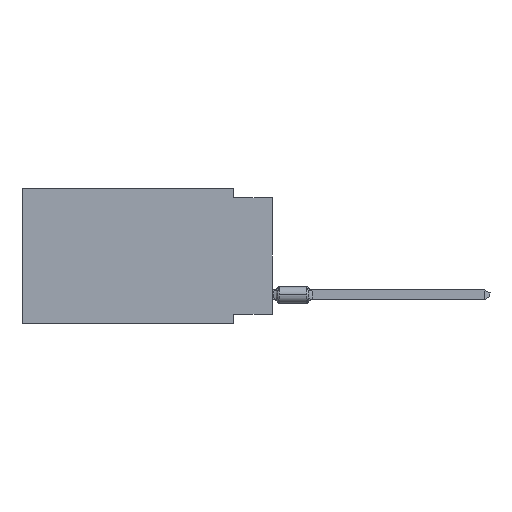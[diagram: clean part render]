
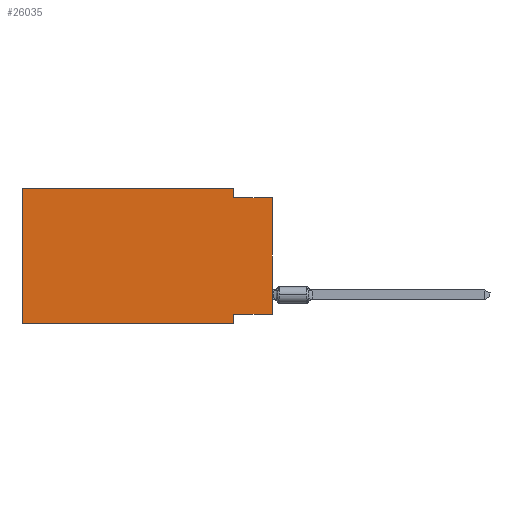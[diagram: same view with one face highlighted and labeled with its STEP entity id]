
A CAD part, left-side view. The second image highlights one B-rep face of the part: STEP entity #26035.
In plain terms, the highlighted planar face has unit normal (-1, 0, 0).
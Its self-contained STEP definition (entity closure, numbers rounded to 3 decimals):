
#2601 = CARTESIAN_POINT ( 'NONE',  ( 0., 16.383, 0. ) ) ;
#3043 = DIRECTION ( 'NONE',  ( 0., 0., 1. ) ) ;
#3452 = DIRECTION ( 'NONE',  ( 0., -1., 0. ) ) ;
#3476 = LINE ( 'NONE', #7590, #48642 ) ;
#3518 = LINE ( 'NONE', #36686, #8659 ) ;
#3585 = VERTEX_POINT ( 'NONE', #44069 ) ;
#4729 = VERTEX_POINT ( 'NONE', #6544 ) ;
#5731 = ORIENTED_EDGE ( 'NONE', *, *, #37576, .F. ) ;
#6544 = CARTESIAN_POINT ( 'NONE',  ( 0., 16.383, -8.89 ) ) ;
#6561 = AXIS2_PLACEMENT_3D ( 'NONE', #48879, #20068, #49409 ) ;
#7590 = CARTESIAN_POINT ( 'NONE',  ( 0., 16.383, -8.89 ) ) ;
#7794 = LINE ( 'NONE', #2601, #51098 ) ;
#8154 = ORIENTED_EDGE ( 'NONE', *, *, #47848, .F. ) ;
#8659 = VECTOR ( 'NONE', #41069, 1000. ) ;
#9269 = ORIENTED_EDGE ( 'NONE', *, *, #39718, .F. ) ;
#9792 = LINE ( 'NONE', #44754, #15389 ) ;
#10535 = ORIENTED_EDGE ( 'NONE', *, *, #14698, .F. ) ;
#11265 = LINE ( 'NONE', #19460, #43617 ) ;
#11359 = DIRECTION ( 'NONE',  ( 0., -1., 0. ) ) ;
#11933 = CARTESIAN_POINT ( 'NONE',  ( 0., 0., -0.635 ) ) ;
#14216 = VERTEX_POINT ( 'NONE', #29497 ) ;
#14698 = EDGE_CURVE ( 'NONE', #32085, #25945, #36820, .T. ) ;
#14884 = DIRECTION ( 'NONE',  ( 0., 0., -1. ) ) ;
#15023 = ORIENTED_EDGE ( 'NONE', *, *, #52276, .F. ) ;
#15389 = VECTOR ( 'NONE', #14884, 1000. ) ;
#16014 = CARTESIAN_POINT ( 'NONE',  ( 0., 2.54, -8.89 ) ) ;
#16252 = ORIENTED_EDGE ( 'NONE', *, *, #40218, .F. ) ;
#17627 = DIRECTION ( 'NONE',  ( 0., 0., 1. ) ) ;
#17725 = VECTOR ( 'NONE', #29119, 1000. ) ;
#19460 = CARTESIAN_POINT ( 'NONE',  ( 0., 16.383, 0. ) ) ;
#19691 = ORIENTED_EDGE ( 'NONE', *, *, #44453, .T. ) ;
#20068 = DIRECTION ( 'NONE',  ( 1., 0., 0. ) ) ;
#20894 = VERTEX_POINT ( 'NONE', #16014 ) ;
#22002 = LINE ( 'NONE', #51358, #38965 ) ;
#22058 = VERTEX_POINT ( 'NONE', #44297 ) ;
#23468 = ORIENTED_EDGE ( 'NONE', *, *, #46355, .T. ) ;
#24189 = VECTOR ( 'NONE', #3452, 1000. ) ;
#24281 = LINE ( 'NONE', #11933, #24189 ) ;
#24557 = DIRECTION ( 'NONE',  ( 0., -1., 0. ) ) ;
#25945 = VERTEX_POINT ( 'NONE', #52438 ) ;
#26035 = ADVANCED_FACE ( 'NONE', ( #40641 ), #53253, .F. ) ;
#26358 = CARTESIAN_POINT ( 'NONE',  ( 0., 2.54, 0. ) ) ;
#27156 = VERTEX_POINT ( 'NONE', #53345 ) ;
#29119 = DIRECTION ( 'NONE',  ( 0., 0., -1. ) ) ;
#29497 = CARTESIAN_POINT ( 'NONE',  ( 0., 2.54, -8.255 ) ) ;
#32085 = VERTEX_POINT ( 'NONE', #26358 ) ;
#36686 = CARTESIAN_POINT ( 'NONE',  ( 0., 0., -8.255 ) ) ;
#36820 = LINE ( 'NONE', #37627, #17725 ) ;
#37576 = EDGE_CURVE ( 'NONE', #25945, #22058, #24281, .T. ) ;
#37627 = CARTESIAN_POINT ( 'NONE',  ( 0., 2.54, 0. ) ) ;
#38965 = VECTOR ( 'NONE', #17627, 1000. ) ;
#39718 = EDGE_CURVE ( 'NONE', #4729, #3585, #11265, .T. ) ;
#40218 = EDGE_CURVE ( 'NONE', #27156, #14216, #3518, .T. ) ;
#40641 = FACE_OUTER_BOUND ( 'NONE', #43732, .T. ) ;
#41069 = DIRECTION ( 'NONE',  ( 0., 1., 0. ) ) ;
#43617 = VECTOR ( 'NONE', #3043, 1000. ) ;
#43732 = EDGE_LOOP ( 'NONE', ( #19691, #5731, #10535, #8154, #9269, #23468, #15023, #16252 ) ) ;
#44069 = CARTESIAN_POINT ( 'NONE',  ( 0., 16.383, 0. ) ) ;
#44297 = CARTESIAN_POINT ( 'NONE',  ( 0., 0., -0.635 ) ) ;
#44453 = EDGE_CURVE ( 'NONE', #27156, #22058, #22002, .T. ) ;
#44754 = CARTESIAN_POINT ( 'NONE',  ( 0., 2.54, -8.89 ) ) ;
#46355 = EDGE_CURVE ( 'NONE', #4729, #20894, #3476, .T. ) ;
#47848 = EDGE_CURVE ( 'NONE', #3585, #32085, #7794, .T. ) ;
#48642 = VECTOR ( 'NONE', #24557, 1000. ) ;
#48879 = CARTESIAN_POINT ( 'NONE',  ( 0., 16.383, 0. ) ) ;
#49409 = DIRECTION ( 'NONE',  ( 0., 0., -1. ) ) ;
#51098 = VECTOR ( 'NONE', #11359, 1000. ) ;
#51358 = CARTESIAN_POINT ( 'NONE',  ( 0., 0., 0. ) ) ;
#52276 = EDGE_CURVE ( 'NONE', #14216, #20894, #9792, .T. ) ;
#52438 = CARTESIAN_POINT ( 'NONE',  ( 0., 2.54, -0.635 ) ) ;
#53253 = PLANE ( 'NONE',  #6561 ) ;
#53345 = CARTESIAN_POINT ( 'NONE',  ( 0., 0., -8.255 ) ) ;
